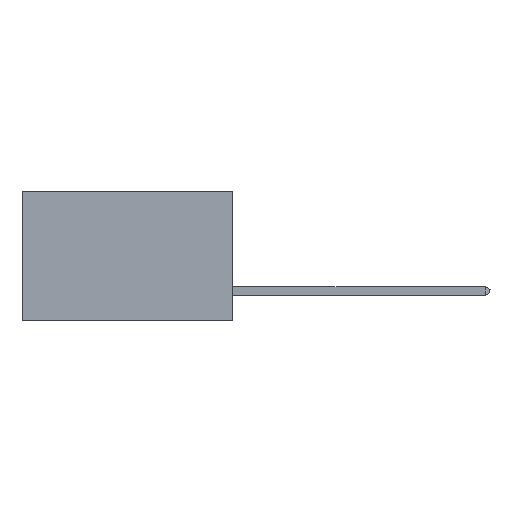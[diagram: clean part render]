
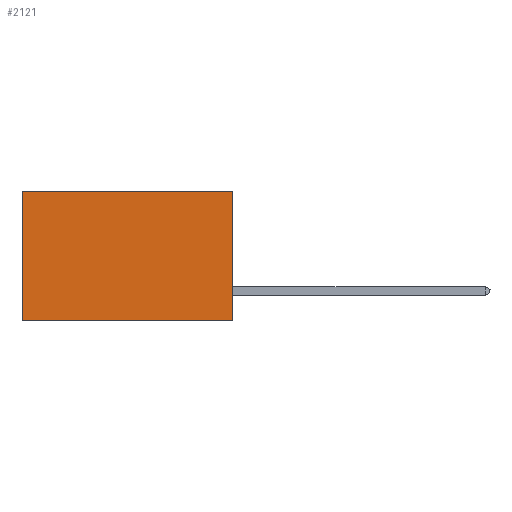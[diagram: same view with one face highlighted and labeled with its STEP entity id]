
A CAD part, left-side view. The second image highlights one B-rep face of the part: STEP entity #2121.
In plain terms, the highlighted planar face has unit normal (-1, 0, 0).
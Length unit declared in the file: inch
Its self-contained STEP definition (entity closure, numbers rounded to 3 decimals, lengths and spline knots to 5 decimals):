
#133 = ORIENTED_EDGE ( 'NONE', *, *, #17955, .T. ) ;
#672 = EDGE_CURVE ( 'NONE', #16577, #2777, #15916, .T. ) ;
#2121 = ADVANCED_FACE ( 'NONE', ( #22464 ), #20891, .F. ) ;
#2759 = VECTOR ( 'NONE', #3928, 39.37008 ) ;
#2777 = VERTEX_POINT ( 'NONE', #10427 ) ;
#2793 = EDGE_LOOP ( 'NONE', ( #133, #12827, #10789, #23800 ) ) ;
#3928 = DIRECTION ( 'NONE',  ( 0., 0., -1. ) ) ;
#4866 = CARTESIAN_POINT ( 'NONE',  ( 0.2875, 0., 0. ) ) ;
#8724 = LINE ( 'NONE', #4866, #24241 ) ;
#8730 = DIRECTION ( 'NONE',  ( 1., 0., 0. ) ) ;
#8789 = EDGE_CURVE ( 'NONE', #11390, #16577, #8724, .T. ) ;
#9862 = VECTOR ( 'NONE', #10917, 39.37008 ) ;
#9971 = CARTESIAN_POINT ( 'NONE',  ( 0.2875, 0.6, 0. ) ) ;
#10427 = CARTESIAN_POINT ( 'NONE',  ( 0.2875, 0.6, -0.37 ) ) ;
#10789 = ORIENTED_EDGE ( 'NONE', *, *, #8789, .F. ) ;
#10917 = DIRECTION ( 'NONE',  ( 0., 1., 0. ) ) ;
#11390 = VERTEX_POINT ( 'NONE', #19315 ) ;
#12217 = CARTESIAN_POINT ( 'NONE',  ( 0.2875, 0., -0.37 ) ) ;
#12625 = CARTESIAN_POINT ( 'NONE',  ( 0.2875, 0., 0. ) ) ;
#12827 = ORIENTED_EDGE ( 'NONE', *, *, #672, .F. ) ;
#14860 = LINE ( 'NONE', #9971, #2759 ) ;
#14864 = VERTEX_POINT ( 'NONE', #25476 ) ;
#15916 = LINE ( 'NONE', #18667, #9862 ) ;
#16577 = VERTEX_POINT ( 'NONE', #12217 ) ;
#16601 = VECTOR ( 'NONE', #24834, 39.37008 ) ;
#16801 = DIRECTION ( 'NONE',  ( 0., 0., -1. ) ) ;
#17955 = EDGE_CURVE ( 'NONE', #14864, #2777, #14860, .T. ) ;
#18667 = CARTESIAN_POINT ( 'NONE',  ( 0.2875, 0., -0.37 ) ) ;
#18980 = AXIS2_PLACEMENT_3D ( 'NONE', #21149, #8730, #23094 ) ;
#19315 = CARTESIAN_POINT ( 'NONE',  ( 0.2875, 0., 0. ) ) ;
#20803 = EDGE_CURVE ( 'NONE', #11390, #14864, #25121, .T. ) ;
#20891 = PLANE ( 'NONE',  #18980 ) ;
#21149 = CARTESIAN_POINT ( 'NONE',  ( 0.2875, 0., 0. ) ) ;
#22464 = FACE_OUTER_BOUND ( 'NONE', #2793, .T. ) ;
#23094 = DIRECTION ( 'NONE',  ( 0., 0., -1. ) ) ;
#23800 = ORIENTED_EDGE ( 'NONE', *, *, #20803, .T. ) ;
#24241 = VECTOR ( 'NONE', #16801, 39.37008 ) ;
#24834 = DIRECTION ( 'NONE',  ( 0., 1., 0. ) ) ;
#25121 = LINE ( 'NONE', #12625, #16601 ) ;
#25476 = CARTESIAN_POINT ( 'NONE',  ( 0.2875, 0.6, 0. ) ) ;
